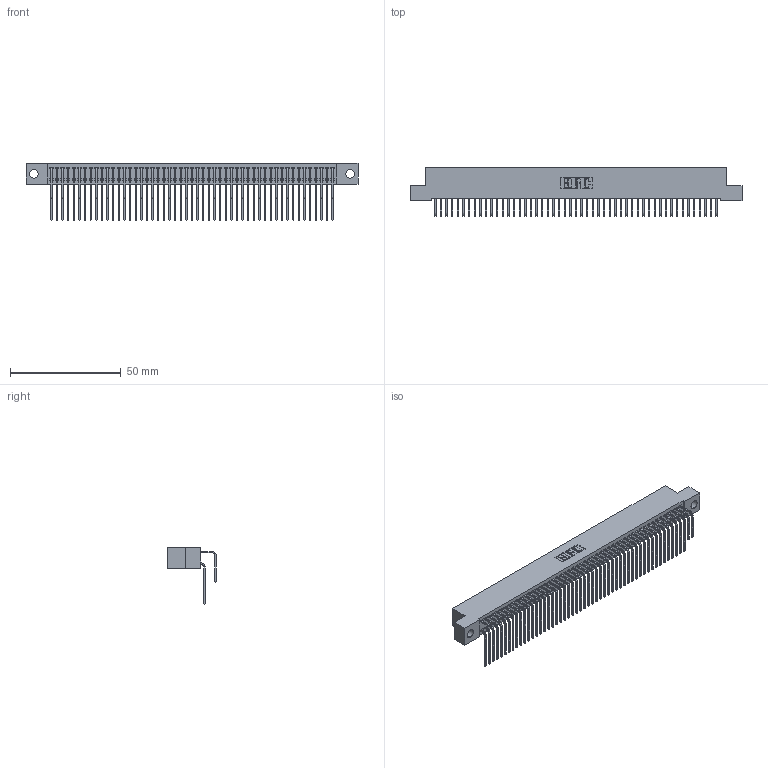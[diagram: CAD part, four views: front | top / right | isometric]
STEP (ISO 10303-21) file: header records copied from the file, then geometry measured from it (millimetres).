
FILE_DESCRIPTION (( 'STEP AP203' ), '1' );
FILE_NAME ('342-102-558-204.STEP', '2019-10-04T18:22:22', ( '' ), ( '' ), 'SwSTEP 2.0', 'SolidWorks 2016', '' );
FILE_SCHEMA (( 'CONFIG_CONTROL_DESIGN' ));
Length unit declared in the file: inch
Products named in the file (4): 345-292-001_558 559 Tail - 1; 345-292-001_558 Tail - 2; 342-102-558-204; 342 Part_.156 TH
Assembly tree (103 placements, depth 2):
  342-102-558-204
    342 Part_.156 TH
    345-292-001_558 559 Tail - 1  x51
    345-292-001_558 Tail - 2  x51
Bounding box: 149.86 x 21.91 x 25.78 mm (x, y, z)
Volume: 14008.9 mm3; surface area: 25510.7 mm2
Topology: 103 solids, 103 shells, 5618 faces, 16721 edges, 11010 vertices
Faces by surface type: plane 3942, cylinder 1676
Entity records: 33301 total; most frequent: CARTESIAN_POINT 5557, ORIENTED_EDGE 5442, DIRECTION 4713, EDGE_CURVE 2721, VECTOR 2553, LINE 2553, VERTEX_POINT 1810, AXIS2_PLACEMENT_3D 1080
